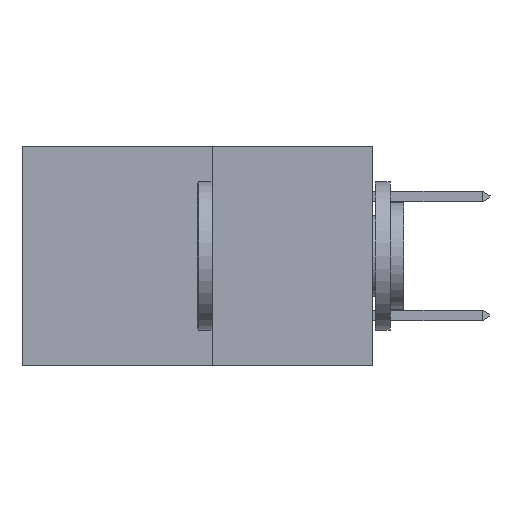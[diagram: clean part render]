
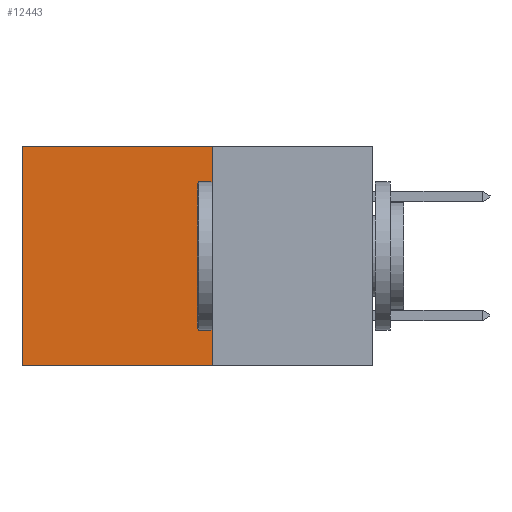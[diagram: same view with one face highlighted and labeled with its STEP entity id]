
A CAD part, left-side view. The second image highlights one B-rep face of the part: STEP entity #12443.
In plain terms, the highlighted planar face has unit normal (-1, 0, 0).
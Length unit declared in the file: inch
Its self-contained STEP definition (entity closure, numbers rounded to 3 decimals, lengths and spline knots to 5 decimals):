
#264 = AXIS2_PLACEMENT_3D ( 'NONE', #15199, #14125, #7211 ) ;
#544 = LINE ( 'NONE', #8677, #9864 ) ;
#1013 = VECTOR ( 'NONE', #8771, 39.37008 ) ;
#1479 = CARTESIAN_POINT ( 'NONE',  ( 0.277, 0.27, 0. ) ) ;
#2269 = VECTOR ( 'NONE', #7227, 39.37008 ) ;
#2663 = LINE ( 'NONE', #1479, #14352 ) ;
#3146 = FACE_OUTER_BOUND ( 'NONE', #5558, .T. ) ;
#3339 = CARTESIAN_POINT ( 'NONE',  ( 0.277, 0.59, -0.37 ) ) ;
#3516 = VERTEX_POINT ( 'NONE', #3339 ) ;
#3522 = ORIENTED_EDGE ( 'NONE', *, *, #8793, .T. ) ;
#4496 = VERTEX_POINT ( 'NONE', #6297 ) ;
#5082 = VERTEX_POINT ( 'NONE', #6314 ) ;
#5548 = ORIENTED_EDGE ( 'NONE', *, *, #15129, .T. ) ;
#5558 = EDGE_LOOP ( 'NONE', ( #3522, #7536, #9713, #5548 ) ) ;
#6293 = CARTESIAN_POINT ( 'NONE',  ( 0.277, 0.59, 0. ) ) ;
#6297 = CARTESIAN_POINT ( 'NONE',  ( 0.277, 0.27, 0. ) ) ;
#6314 = CARTESIAN_POINT ( 'NONE',  ( 0.277, 0.27, -0.37 ) ) ;
#7211 = DIRECTION ( 'NONE',  ( 0., 0., -1. ) ) ;
#7227 = DIRECTION ( 'NONE',  ( 0., 1., 0. ) ) ;
#7492 = LINE ( 'NONE', #8968, #1013 ) ;
#7536 = ORIENTED_EDGE ( 'NONE', *, *, #13775, .F. ) ;
#8659 = DIRECTION ( 'NONE',  ( 0., 0., -1. ) ) ;
#8677 = CARTESIAN_POINT ( 'NONE',  ( 0.277, 0.27, -0.37 ) ) ;
#8771 = DIRECTION ( 'NONE',  ( 0., 0., -1. ) ) ;
#8793 = EDGE_CURVE ( 'NONE', #15080, #3516, #7492, .T. ) ;
#8968 = CARTESIAN_POINT ( 'NONE',  ( 0.277, 0.59, -0.37 ) ) ;
#9713 = ORIENTED_EDGE ( 'NONE', *, *, #10174, .F. ) ;
#9864 = VECTOR ( 'NONE', #8659, 39.37008 ) ;
#10174 = EDGE_CURVE ( 'NONE', #4496, #5082, #544, .T. ) ;
#11043 = DIRECTION ( 'NONE',  ( 0., 1., 0. ) ) ;
#12443 = ADVANCED_FACE ( 'NONE', ( #3146 ), #13005, .F. ) ;
#13005 = PLANE ( 'NONE',  #264 ) ;
#13775 = EDGE_CURVE ( 'NONE', #5082, #3516, #14716, .T. ) ;
#14125 = DIRECTION ( 'NONE',  ( 1., 0., 0. ) ) ;
#14187 = CARTESIAN_POINT ( 'NONE',  ( 0.277, 0.27, -0.37 ) ) ;
#14352 = VECTOR ( 'NONE', #11043, 39.37008 ) ;
#14716 = LINE ( 'NONE', #14187, #2269 ) ;
#15080 = VERTEX_POINT ( 'NONE', #6293 ) ;
#15129 = EDGE_CURVE ( 'NONE', #4496, #15080, #2663, .T. ) ;
#15199 = CARTESIAN_POINT ( 'NONE',  ( 0.277, 0.27, -0.37 ) ) ;
